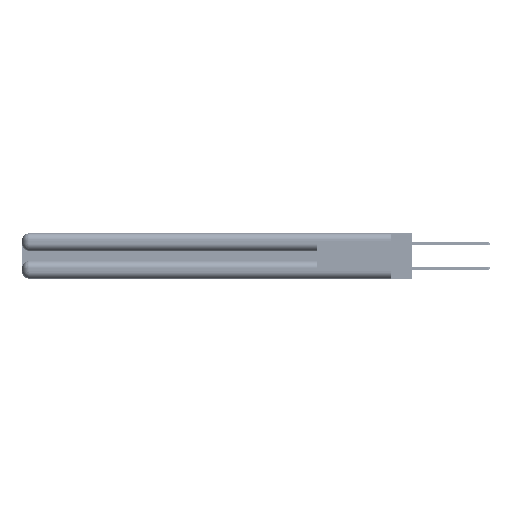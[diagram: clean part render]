
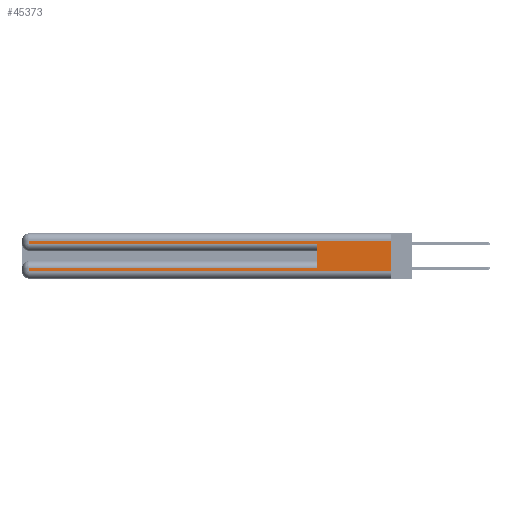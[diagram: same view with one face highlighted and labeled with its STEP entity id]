
A CAD part, left-side view. The second image highlights one B-rep face of the part: STEP entity #45373.
In plain terms, the highlighted planar face has unit normal (-1, 0, 0).
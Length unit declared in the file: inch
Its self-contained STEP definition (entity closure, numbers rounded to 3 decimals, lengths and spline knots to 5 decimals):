
#779 = VECTOR ( 'NONE', #4776, 39.37008 ) ;
#1446 = LINE ( 'NONE', #34073, #50796 ) ;
#2618 = CARTESIAN_POINT ( 'NONE',  ( 0., 0.6, 0.145 ) ) ;
#3862 = DIRECTION ( 'NONE',  ( 0., 1., 0. ) ) ;
#3930 = DIRECTION ( 'NONE',  ( 0., -1., 0. ) ) ;
#4776 = DIRECTION ( 'NONE',  ( 0., 1., 0. ) ) ;
#4966 = LINE ( 'NONE', #7989, #22319 ) ;
#5030 = LINE ( 'NONE', #38919, #47002 ) ;
#5477 = EDGE_LOOP ( 'NONE', ( #38453, #16162, #37698, #30725, #8601, #42341, #49779, #46672 ) ) ;
#6031 = EDGE_CURVE ( 'NONE', #25418, #26149, #34828, .T. ) ;
#6623 = VERTEX_POINT ( 'NONE', #11484 ) ;
#6743 = VERTEX_POINT ( 'NONE', #8439 ) ;
#7383 = CARTESIAN_POINT ( 'NONE',  ( 0., 0.6, 0.285 ) ) ;
#7989 = CARTESIAN_POINT ( 'NONE',  ( 0., 0., 0.085 ) ) ;
#8439 = CARTESIAN_POINT ( 'NONE',  ( 0., 0.6, 0.085 ) ) ;
#8601 = ORIENTED_EDGE ( 'NONE', *, *, #21832, .F. ) ;
#8724 = DIRECTION ( 'NONE',  ( 0., -1., 0. ) ) ;
#9320 = CARTESIAN_POINT ( 'NONE',  ( 0., 2.94, 0.285 ) ) ;
#9362 = EDGE_CURVE ( 'NONE', #6623, #30343, #37412, .T. ) ;
#11484 = CARTESIAN_POINT ( 'NONE',  ( 0., 2.94, 0.085 ) ) ;
#14570 = VECTOR ( 'NONE', #32442, 39.37008 ) ;
#14918 = DIRECTION ( 'NONE',  ( 0., 0., -1. ) ) ;
#15771 = LINE ( 'NONE', #18998, #41804 ) ;
#15911 = VERTEX_POINT ( 'NONE', #7383 ) ;
#16162 = ORIENTED_EDGE ( 'NONE', *, *, #6031, .T. ) ;
#16969 = PLANE ( 'NONE',  #30638 ) ;
#18998 = CARTESIAN_POINT ( 'NONE',  ( 0., 2.94, 0.37 ) ) ;
#20533 = LINE ( 'NONE', #2618, #14570 ) ;
#20542 = CARTESIAN_POINT ( 'NONE',  ( 0., 0., 0.06 ) ) ;
#21832 = EDGE_CURVE ( 'NONE', #6743, #15911, #20533, .T. ) ;
#22319 = VECTOR ( 'NONE', #3862, 39.37008 ) ;
#22636 = CARTESIAN_POINT ( 'NONE',  ( 0., 2.94, 0.37 ) ) ;
#25418 = VERTEX_POINT ( 'NONE', #34029 ) ;
#26149 = VERTEX_POINT ( 'NONE', #34333 ) ;
#26544 = DIRECTION ( 'NONE',  ( 0., 0., -1. ) ) ;
#26746 = LINE ( 'NONE', #20542, #54050 ) ;
#27307 = VERTEX_POINT ( 'NONE', #38876 ) ;
#27648 = CARTESIAN_POINT ( 'NONE',  ( 0., 2.94, 0.06 ) ) ;
#29638 = DIRECTION ( 'NONE',  ( 0., 0., -1. ) ) ;
#30343 = VERTEX_POINT ( 'NONE', #27648 ) ;
#30590 = EDGE_CURVE ( 'NONE', #30343, #27307, #26746, .T. ) ;
#30638 = AXIS2_PLACEMENT_3D ( 'NONE', #50705, #54994, #29638 ) ;
#30725 = ORIENTED_EDGE ( 'NONE', *, *, #40842, .T. ) ;
#30889 = DIRECTION ( 'NONE',  ( 0., 0., -1. ) ) ;
#32442 = DIRECTION ( 'NONE',  ( 0., 0., 1. ) ) ;
#33810 = FACE_OUTER_BOUND ( 'NONE', #5477, .T. ) ;
#34029 = CARTESIAN_POINT ( 'NONE',  ( 0., 0., 0.31 ) ) ;
#34073 = CARTESIAN_POINT ( 'NONE',  ( 0., 0., 0.37 ) ) ;
#34333 = CARTESIAN_POINT ( 'NONE',  ( 0., 2.94, 0.31 ) ) ;
#34828 = LINE ( 'NONE', #54904, #779 ) ;
#37412 = LINE ( 'NONE', #22636, #41427 ) ;
#37698 = ORIENTED_EDGE ( 'NONE', *, *, #45865, .T. ) ;
#38453 = ORIENTED_EDGE ( 'NONE', *, *, #51670, .F. ) ;
#38876 = CARTESIAN_POINT ( 'NONE',  ( 0., 0., 0.06 ) ) ;
#38919 = CARTESIAN_POINT ( 'NONE',  ( 0., 0., 0.285 ) ) ;
#40739 = EDGE_CURVE ( 'NONE', #6743, #6623, #4966, .T. ) ;
#40842 = EDGE_CURVE ( 'NONE', #43471, #15911, #5030, .T. ) ;
#41427 = VECTOR ( 'NONE', #26544, 39.37008 ) ;
#41804 = VECTOR ( 'NONE', #14918, 39.37008 ) ;
#42341 = ORIENTED_EDGE ( 'NONE', *, *, #40739, .T. ) ;
#43471 = VERTEX_POINT ( 'NONE', #9320 ) ;
#45373 = ADVANCED_FACE ( 'NONE', ( #33810 ), #16969, .F. ) ;
#45865 = EDGE_CURVE ( 'NONE', #26149, #43471, #15771, .T. ) ;
#46672 = ORIENTED_EDGE ( 'NONE', *, *, #30590, .T. ) ;
#47002 = VECTOR ( 'NONE', #8724, 39.37008 ) ;
#49779 = ORIENTED_EDGE ( 'NONE', *, *, #9362, .T. ) ;
#50705 = CARTESIAN_POINT ( 'NONE',  ( 0., 0., 0.37 ) ) ;
#50796 = VECTOR ( 'NONE', #30889, 39.37008 ) ;
#51670 = EDGE_CURVE ( 'NONE', #25418, #27307, #1446, .T. ) ;
#54050 = VECTOR ( 'NONE', #3930, 39.37008 ) ;
#54904 = CARTESIAN_POINT ( 'NONE',  ( 0., 0., 0.31 ) ) ;
#54994 = DIRECTION ( 'NONE',  ( 1., 0., 0. ) ) ;
